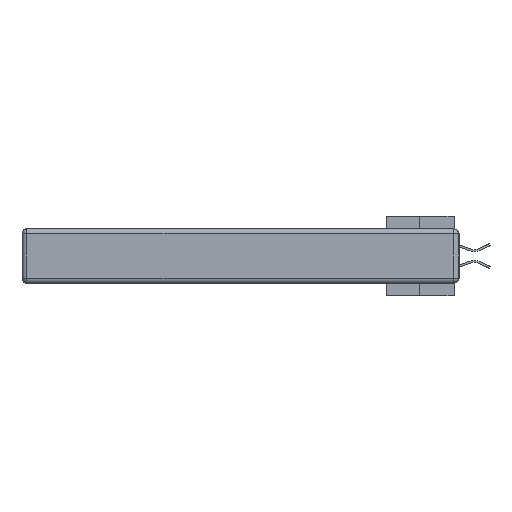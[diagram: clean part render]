
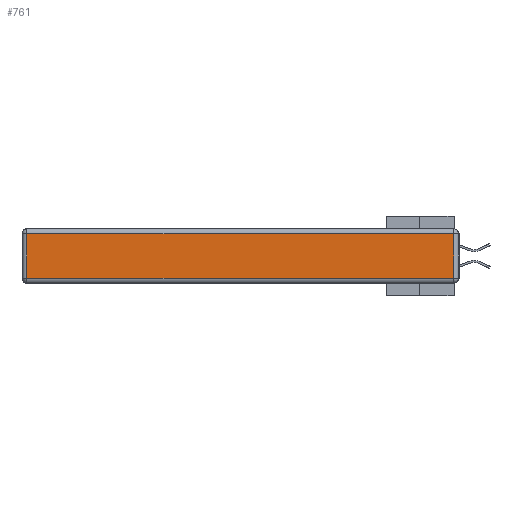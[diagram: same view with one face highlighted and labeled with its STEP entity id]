
A CAD part, left-side view. The second image highlights one B-rep face of the part: STEP entity #761.
In plain terms, the highlighted planar face has unit normal (-1, 0, 0).
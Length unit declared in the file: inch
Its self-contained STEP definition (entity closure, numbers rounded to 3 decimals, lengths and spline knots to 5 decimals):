
#199 = CARTESIAN_POINT ( 'NONE',  ( 0., 0.03, -0.03 ) ) ;
#761 = ADVANCED_FACE ( 'NONE', ( #7139 ), #31086, .T. ) ;
#2147 = DIRECTION ( 'NONE',  ( 0., 0., -1. ) ) ;
#2234 = EDGE_CURVE ( 'NONE', #38569, #20142, #13315, .T. ) ;
#3936 = VECTOR ( 'NONE', #7660, 39.37008 ) ;
#5350 = EDGE_CURVE ( 'NONE', #37554, #18941, #9673, .T. ) ;
#7139 = FACE_OUTER_BOUND ( 'NONE', #24276, .T. ) ;
#7660 = DIRECTION ( 'NONE',  ( 0., 0., 1. ) ) ;
#9651 = CARTESIAN_POINT ( 'NONE',  ( 0., 0.03, -0.313 ) ) ;
#9673 = LINE ( 'NONE', #18574, #25058 ) ;
#10577 = EDGE_CURVE ( 'NONE', #18941, #38569, #19372, .T. ) ;
#12592 = CARTESIAN_POINT ( 'NONE',  ( 0., 2.72, -0.03 ) ) ;
#12708 = CARTESIAN_POINT ( 'NONE',  ( 0., 0., -0.343 ) ) ;
#13315 = LINE ( 'NONE', #17128, #35437 ) ;
#14105 = LINE ( 'NONE', #14387, #36712 ) ;
#14387 = CARTESIAN_POINT ( 'NONE',  ( 0., 2.72, -0.343 ) ) ;
#15178 = DIRECTION ( 'NONE',  ( 0., -1., 0. ) ) ;
#15921 = EDGE_CURVE ( 'NONE', #20142, #37554, #14105, .T. ) ;
#16543 = ORIENTED_EDGE ( 'NONE', *, *, #5350, .T. ) ;
#17128 = CARTESIAN_POINT ( 'NONE',  ( 0., 2.75, -0.03 ) ) ;
#17198 = CARTESIAN_POINT ( 'NONE',  ( 0., 2.72, -0.313 ) ) ;
#18241 = AXIS2_PLACEMENT_3D ( 'NONE', #12708, #37275, #18925 ) ;
#18574 = CARTESIAN_POINT ( 'NONE',  ( 0., 0., -0.313 ) ) ;
#18925 = DIRECTION ( 'NONE',  ( 0., 0., 1. ) ) ;
#18941 = VERTEX_POINT ( 'NONE', #9651 ) ;
#19372 = LINE ( 'NONE', #26071, #3936 ) ;
#20142 = VERTEX_POINT ( 'NONE', #12592 ) ;
#24276 = EDGE_LOOP ( 'NONE', ( #16543, #32564, #27942, #32771 ) ) ;
#25058 = VECTOR ( 'NONE', #15178, 39.37008 ) ;
#26071 = CARTESIAN_POINT ( 'NONE',  ( 0., 0.03, -0.343 ) ) ;
#26756 = DIRECTION ( 'NONE',  ( 0., 1., 0. ) ) ;
#27942 = ORIENTED_EDGE ( 'NONE', *, *, #2234, .T. ) ;
#31086 = PLANE ( 'NONE',  #18241 ) ;
#32564 = ORIENTED_EDGE ( 'NONE', *, *, #10577, .T. ) ;
#32771 = ORIENTED_EDGE ( 'NONE', *, *, #15921, .T. ) ;
#35437 = VECTOR ( 'NONE', #26756, 39.37008 ) ;
#36712 = VECTOR ( 'NONE', #2147, 39.37008 ) ;
#37275 = DIRECTION ( 'NONE',  ( -1., 0., 0. ) ) ;
#37554 = VERTEX_POINT ( 'NONE', #17198 ) ;
#38569 = VERTEX_POINT ( 'NONE', #199 ) ;
